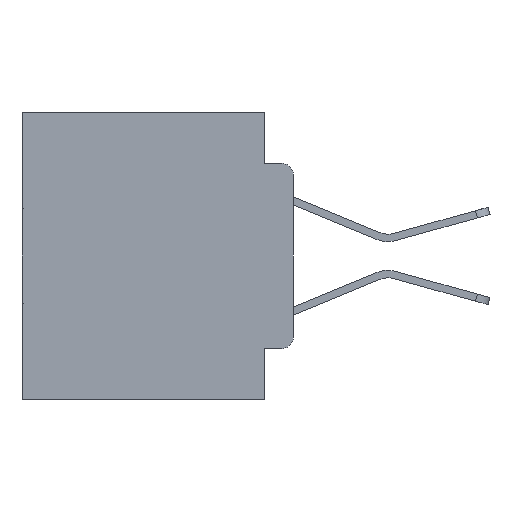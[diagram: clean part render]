
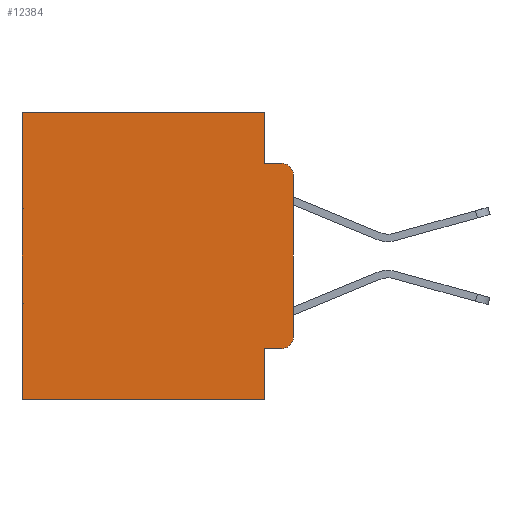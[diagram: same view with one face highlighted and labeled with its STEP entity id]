
A CAD part, left-side view. The second image highlights one B-rep face of the part: STEP entity #12384.
In plain terms, the highlighted planar face has unit normal (-1, 0, 0).
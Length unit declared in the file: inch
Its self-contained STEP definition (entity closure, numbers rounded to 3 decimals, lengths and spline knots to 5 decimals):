
#91 = CIRCLE ( 'NONE', #11212, 0.02 ) ;
#835 = VERTEX_POINT ( 'NONE', #1165 ) ;
#879 = VERTEX_POINT ( 'NONE', #23319 ) ;
#972 = CARTESIAN_POINT ( 'NONE',  ( 0.298, 0.473, -0.5 ) ) ;
#1165 = CARTESIAN_POINT ( 'NONE',  ( 0.298, 0., -0.1085 ) ) ;
#1757 = DIRECTION ( 'NONE',  ( 0., 0., -1. ) ) ;
#1778 = DIRECTION ( 'NONE',  ( -1., 0., 0. ) ) ;
#2803 = CARTESIAN_POINT ( 'NONE',  ( 0.298, 0.051, 0. ) ) ;
#2997 = VERTEX_POINT ( 'NONE', #9133 ) ;
#3791 = LINE ( 'NONE', #22338, #15707 ) ;
#4459 = AXIS2_PLACEMENT_3D ( 'NONE', #16105, #1778, #18474 ) ;
#4862 = LINE ( 'NONE', #30023, #29062 ) ;
#6601 = CARTESIAN_POINT ( 'NONE',  ( 0.298, 0., 0. ) ) ;
#7115 = CARTESIAN_POINT ( 'NONE',  ( 0.298, 0.473, 0. ) ) ;
#7188 = ORIENTED_EDGE ( 'NONE', *, *, #8237, .F. ) ;
#7931 = ORIENTED_EDGE ( 'NONE', *, *, #20789, .F. ) ;
#7981 = VERTEX_POINT ( 'NONE', #14772 ) ;
#8139 = CARTESIAN_POINT ( 'NONE',  ( 0.298, 0.473, 0. ) ) ;
#8237 = EDGE_CURVE ( 'NONE', #835, #7981, #21528, .T. ) ;
#8873 = DIRECTION ( 'NONE',  ( 0., -1., 0. ) ) ;
#8910 = CARTESIAN_POINT ( 'NONE',  ( 0.298, 0.051, -0.5 ) ) ;
#8952 = ORIENTED_EDGE ( 'NONE', *, *, #23959, .T. ) ;
#9088 = VECTOR ( 'NONE', #13299, 39.37008 ) ;
#9105 = DIRECTION ( 'NONE',  ( 0., 0., -1. ) ) ;
#9133 = CARTESIAN_POINT ( 'NONE',  ( 0.298, 0.02, -0.0885 ) ) ;
#9205 = FACE_OUTER_BOUND ( 'NONE', #24545, .T. ) ;
#9340 = CIRCLE ( 'NONE', #4459, 0.02 ) ;
#9494 = DIRECTION ( 'NONE',  ( 0., 1., 0. ) ) ;
#9772 = ORIENTED_EDGE ( 'NONE', *, *, #10772, .F. ) ;
#9827 = EDGE_CURVE ( 'NONE', #13933, #2997, #23656, .T. ) ;
#10772 = EDGE_CURVE ( 'NONE', #16087, #30620, #19598, .T. ) ;
#10905 = VERTEX_POINT ( 'NONE', #26464 ) ;
#11185 = VECTOR ( 'NONE', #14969, 39.37008 ) ;
#11212 = AXIS2_PLACEMENT_3D ( 'NONE', #14294, #30563, #16667 ) ;
#11376 = EDGE_CURVE ( 'NONE', #835, #2997, #91, .T. ) ;
#11523 = VERTEX_POINT ( 'NONE', #2803 ) ;
#12284 = ORIENTED_EDGE ( 'NONE', *, *, #9827, .F. ) ;
#12384 = ADVANCED_FACE ( 'NONE', ( #9205 ), #25378, .F. ) ;
#12589 = LINE ( 'NONE', #8139, #18094 ) ;
#13299 = DIRECTION ( 'NONE',  ( 0., 0., -1. ) ) ;
#13933 = VERTEX_POINT ( 'NONE', #24172 ) ;
#14294 = CARTESIAN_POINT ( 'NONE',  ( 0.298, 0.02, -0.1085 ) ) ;
#14772 = CARTESIAN_POINT ( 'NONE',  ( 0.298, 0., -0.3915 ) ) ;
#14928 = VERTEX_POINT ( 'NONE', #7115 ) ;
#14969 = DIRECTION ( 'NONE',  ( 0., -1., 0. ) ) ;
#15138 = DIRECTION ( 'NONE',  ( 0., 0., -1. ) ) ;
#15707 = VECTOR ( 'NONE', #27033, 39.37008 ) ;
#16073 = DIRECTION ( 'NONE',  ( 0., 1., 0. ) ) ;
#16086 = DIRECTION ( 'NONE',  ( 1., 0., 0. ) ) ;
#16087 = VERTEX_POINT ( 'NONE', #8910 ) ;
#16105 = CARTESIAN_POINT ( 'NONE',  ( 0.298, 0.02, -0.3915 ) ) ;
#16121 = EDGE_CURVE ( 'NONE', #11523, #13933, #4862, .T. ) ;
#16361 = ORIENTED_EDGE ( 'NONE', *, *, #27068, .T. ) ;
#16667 = DIRECTION ( 'NONE',  ( 0., 0., -1. ) ) ;
#17099 = LINE ( 'NONE', #6601, #28045 ) ;
#17321 = CARTESIAN_POINT ( 'NONE',  ( 0.298, 0.051, -0.0885 ) ) ;
#17692 = EDGE_CURVE ( 'NONE', #14928, #30620, #12589, .T. ) ;
#17787 = ORIENTED_EDGE ( 'NONE', *, *, #17692, .T. ) ;
#18094 = VECTOR ( 'NONE', #15138, 39.37008 ) ;
#18474 = DIRECTION ( 'NONE',  ( 0., 0., -1. ) ) ;
#19598 = LINE ( 'NONE', #25860, #28324 ) ;
#19705 = ORIENTED_EDGE ( 'NONE', *, *, #16121, .F. ) ;
#20419 = ORIENTED_EDGE ( 'NONE', *, *, #11376, .T. ) ;
#20517 = ORIENTED_EDGE ( 'NONE', *, *, #21661, .T. ) ;
#20541 = CARTESIAN_POINT ( 'NONE',  ( 0.298, 0.051, -0.4115 ) ) ;
#20789 = EDGE_CURVE ( 'NONE', #10905, #16087, #3791, .T. ) ;
#21528 = LINE ( 'NONE', #22615, #9088 ) ;
#21661 = EDGE_CURVE ( 'NONE', #11523, #14928, #17099, .T. ) ;
#22338 = CARTESIAN_POINT ( 'NONE',  ( 0.298, 0.051, 0. ) ) ;
#22615 = CARTESIAN_POINT ( 'NONE',  ( 0.298, 0., 0. ) ) ;
#23319 = CARTESIAN_POINT ( 'NONE',  ( 0.298, 0.02, -0.4115 ) ) ;
#23656 = LINE ( 'NONE', #17321, #11185 ) ;
#23848 = VECTOR ( 'NONE', #8873, 39.37008 ) ;
#23959 = EDGE_CURVE ( 'NONE', #879, #7981, #9340, .T. ) ;
#24172 = CARTESIAN_POINT ( 'NONE',  ( 0.298, 0.051, -0.0885 ) ) ;
#24545 = EDGE_LOOP ( 'NONE', ( #7188, #20419, #12284, #19705, #20517, #17787, #9772, #7931, #16361, #8952 ) ) ;
#25295 = LINE ( 'NONE', #20541, #23848 ) ;
#25378 = PLANE ( 'NONE',  #28280 ) ;
#25860 = CARTESIAN_POINT ( 'NONE',  ( 0.298, 0., -0.5 ) ) ;
#26464 = CARTESIAN_POINT ( 'NONE',  ( 0.298, 0.051, -0.4115 ) ) ;
#27033 = DIRECTION ( 'NONE',  ( 0., 0., -1. ) ) ;
#27068 = EDGE_CURVE ( 'NONE', #10905, #879, #25295, .T. ) ;
#28045 = VECTOR ( 'NONE', #16073, 39.37008 ) ;
#28280 = AXIS2_PLACEMENT_3D ( 'NONE', #30016, #16086, #1757 ) ;
#28324 = VECTOR ( 'NONE', #9494, 39.37008 ) ;
#29062 = VECTOR ( 'NONE', #9105, 39.37008 ) ;
#30016 = CARTESIAN_POINT ( 'NONE',  ( 0.298, 0., 0. ) ) ;
#30023 = CARTESIAN_POINT ( 'NONE',  ( 0.298, 0.051, 0. ) ) ;
#30563 = DIRECTION ( 'NONE',  ( -1., 0., 0. ) ) ;
#30620 = VERTEX_POINT ( 'NONE', #972 ) ;
